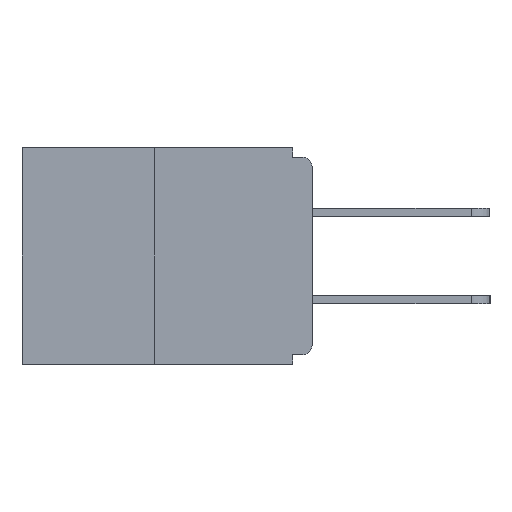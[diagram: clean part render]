
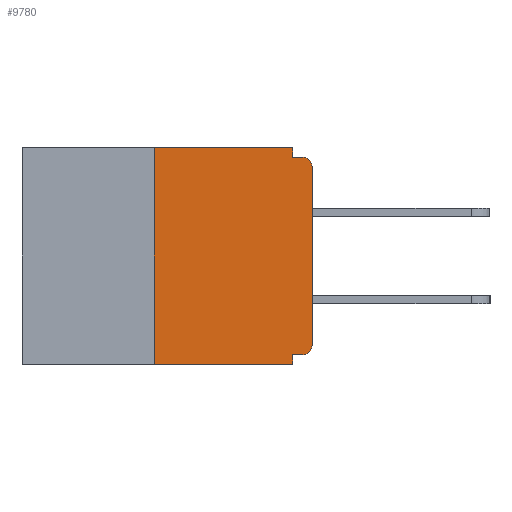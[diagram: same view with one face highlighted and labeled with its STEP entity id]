
A CAD part, left-side view. The second image highlights one B-rep face of the part: STEP entity #9780.
In plain terms, the highlighted planar face has unit normal (-1, 0, 0).
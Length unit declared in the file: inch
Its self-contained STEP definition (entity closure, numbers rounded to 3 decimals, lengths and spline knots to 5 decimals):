
#201 = VERTEX_POINT ( 'NONE', #8685 ) ;
#549 = DIRECTION ( 'NONE',  ( 0., 1., 0. ) ) ;
#617 = CARTESIAN_POINT ( 'NONE',  ( 0., 0.031, -0.015 ) ) ;
#899 = LINE ( 'NONE', #7669, #4076 ) ;
#1092 = EDGE_CURVE ( 'NONE', #4818, #201, #1413, .T. ) ;
#1239 = DIRECTION ( 'NONE',  ( 0., 0., -1. ) ) ;
#1255 = ORIENTED_EDGE ( 'NONE', *, *, #11202, .F. ) ;
#1291 = DIRECTION ( 'NONE',  ( 1., 0., 0. ) ) ;
#1402 = CARTESIAN_POINT ( 'NONE',  ( 0., 0.25, 0. ) ) ;
#1413 = LINE ( 'NONE', #8552, #8360 ) ;
#1423 = CARTESIAN_POINT ( 'NONE',  ( 0., 0.46, -0.343 ) ) ;
#2635 = VERTEX_POINT ( 'NONE', #1402 ) ;
#2672 = VERTEX_POINT ( 'NONE', #9991 ) ;
#2895 = LINE ( 'NONE', #5929, #16191 ) ;
#3040 = ORIENTED_EDGE ( 'NONE', *, *, #1092, .F. ) ;
#3066 = ORIENTED_EDGE ( 'NONE', *, *, #5293, .T. ) ;
#3225 = LINE ( 'NONE', #5891, #10264 ) ;
#3768 = DIRECTION ( 'NONE',  ( -1., 0., 0. ) ) ;
#3902 = DIRECTION ( 'NONE',  ( 0., -1., 0. ) ) ;
#4030 = ORIENTED_EDGE ( 'NONE', *, *, #14993, .T. ) ;
#4072 = EDGE_CURVE ( 'NONE', #9995, #15826, #10538, .T. ) ;
#4076 = VECTOR ( 'NONE', #4929, 39.37008 ) ;
#4242 = DIRECTION ( 'NONE',  ( 0., 0., -1. ) ) ;
#4406 = EDGE_CURVE ( 'NONE', #2672, #2635, #9401, .T. ) ;
#4768 = EDGE_CURVE ( 'NONE', #2635, #13897, #899, .T. ) ;
#4818 = VERTEX_POINT ( 'NONE', #9293 ) ;
#4929 = DIRECTION ( 'NONE',  ( 0., -1., 0. ) ) ;
#5240 = DIRECTION ( 'NONE',  ( 0., 0., -1. ) ) ;
#5293 = EDGE_CURVE ( 'NONE', #16943, #15292, #5437, .T. ) ;
#5437 = CIRCLE ( 'NONE', #14743, 0.015 ) ;
#5603 = ORIENTED_EDGE ( 'NONE', *, *, #6179, .F. ) ;
#5819 = LINE ( 'NONE', #1423, #14019 ) ;
#5891 = CARTESIAN_POINT ( 'NONE',  ( 0., 0., 0. ) ) ;
#5929 = CARTESIAN_POINT ( 'NONE',  ( 0., 0., -0.328 ) ) ;
#6105 = CARTESIAN_POINT ( 'NONE',  ( 0., 0., -0.313 ) ) ;
#6179 = EDGE_CURVE ( 'NONE', #13897, #11870, #12531, .T. ) ;
#6585 = CARTESIAN_POINT ( 'NONE',  ( 0., 0.25, 0. ) ) ;
#6759 = VECTOR ( 'NONE', #3902, 39.37008 ) ;
#6789 = CARTESIAN_POINT ( 'NONE',  ( 0., 0.015, -0.03 ) ) ;
#7179 = ORIENTED_EDGE ( 'NONE', *, *, #4406, .F. ) ;
#7349 = VECTOR ( 'NONE', #4242, 39.37008 ) ;
#7478 = EDGE_CURVE ( 'NONE', #11870, #15292, #16505, .T. ) ;
#7669 = CARTESIAN_POINT ( 'NONE',  ( 0., 0.46, 0. ) ) ;
#7761 = ORIENTED_EDGE ( 'NONE', *, *, #4768, .F. ) ;
#8360 = VECTOR ( 'NONE', #1239, 39.37008 ) ;
#8552 = CARTESIAN_POINT ( 'NONE',  ( 0., 0.031, -0.343 ) ) ;
#8685 = CARTESIAN_POINT ( 'NONE',  ( 0., 0.031, -0.343 ) ) ;
#9293 = CARTESIAN_POINT ( 'NONE',  ( 0., 0.031, -0.328 ) ) ;
#9342 = VECTOR ( 'NONE', #10764, 39.37008 ) ;
#9401 = LINE ( 'NONE', #6585, #9342 ) ;
#9685 = CARTESIAN_POINT ( 'NONE',  ( 0., 0.46, 0. ) ) ;
#9780 = ADVANCED_FACE ( 'NONE', ( #10964 ), #13790, .F. ) ;
#9991 = CARTESIAN_POINT ( 'NONE',  ( 0., 0.25, -0.343 ) ) ;
#9995 = VERTEX_POINT ( 'NONE', #11926 ) ;
#10264 = VECTOR ( 'NONE', #14460, 39.37008 ) ;
#10356 = EDGE_LOOP ( 'NONE', ( #7761, #7179, #10731, #3040, #1255, #16300, #4030, #3066, #13824, #5603 ) ) ;
#10538 = CIRCLE ( 'NONE', #14916, 0.015 ) ;
#10731 = ORIENTED_EDGE ( 'NONE', *, *, #14362, .T. ) ;
#10764 = DIRECTION ( 'NONE',  ( 0., 0., 1. ) ) ;
#10964 = FACE_OUTER_BOUND ( 'NONE', #10356, .T. ) ;
#10987 = CARTESIAN_POINT ( 'NONE',  ( 0., 0.031, 0. ) ) ;
#11202 = EDGE_CURVE ( 'NONE', #9995, #4818, #2895, .T. ) ;
#11870 = VERTEX_POINT ( 'NONE', #617 ) ;
#11926 = CARTESIAN_POINT ( 'NONE',  ( 0., 0.015, -0.328 ) ) ;
#11984 = DIRECTION ( 'NONE',  ( -1., 0., 0. ) ) ;
#12343 = DIRECTION ( 'NONE',  ( 0., 0., -1. ) ) ;
#12419 = DIRECTION ( 'NONE',  ( 0., 0., -1. ) ) ;
#12531 = LINE ( 'NONE', #10987, #7349 ) ;
#12658 = CARTESIAN_POINT ( 'NONE',  ( 0., 0.031, 0. ) ) ;
#13790 = PLANE ( 'NONE',  #13802 ) ;
#13802 = AXIS2_PLACEMENT_3D ( 'NONE', #9685, #1291, #12419 ) ;
#13824 = ORIENTED_EDGE ( 'NONE', *, *, #7478, .F. ) ;
#13897 = VERTEX_POINT ( 'NONE', #12658 ) ;
#14019 = VECTOR ( 'NONE', #16964, 39.37008 ) ;
#14362 = EDGE_CURVE ( 'NONE', #2672, #201, #5819, .T. ) ;
#14460 = DIRECTION ( 'NONE',  ( 0., 0., 1. ) ) ;
#14743 = AXIS2_PLACEMENT_3D ( 'NONE', #6789, #3768, #12343 ) ;
#14916 = AXIS2_PLACEMENT_3D ( 'NONE', #16102, #11984, #5240 ) ;
#14993 = EDGE_CURVE ( 'NONE', #15826, #16943, #3225, .T. ) ;
#15292 = VERTEX_POINT ( 'NONE', #18025 ) ;
#15826 = VERTEX_POINT ( 'NONE', #6105 ) ;
#16102 = CARTESIAN_POINT ( 'NONE',  ( 0., 0.015, -0.313 ) ) ;
#16191 = VECTOR ( 'NONE', #549, 39.37008 ) ;
#16300 = ORIENTED_EDGE ( 'NONE', *, *, #4072, .T. ) ;
#16505 = LINE ( 'NONE', #18061, #6759 ) ;
#16943 = VERTEX_POINT ( 'NONE', #17677 ) ;
#16964 = DIRECTION ( 'NONE',  ( 0., -1., 0. ) ) ;
#17677 = CARTESIAN_POINT ( 'NONE',  ( 0., 0., -0.03 ) ) ;
#18025 = CARTESIAN_POINT ( 'NONE',  ( 0., 0.015, -0.015 ) ) ;
#18061 = CARTESIAN_POINT ( 'NONE',  ( 0., 0., -0.015 ) ) ;
